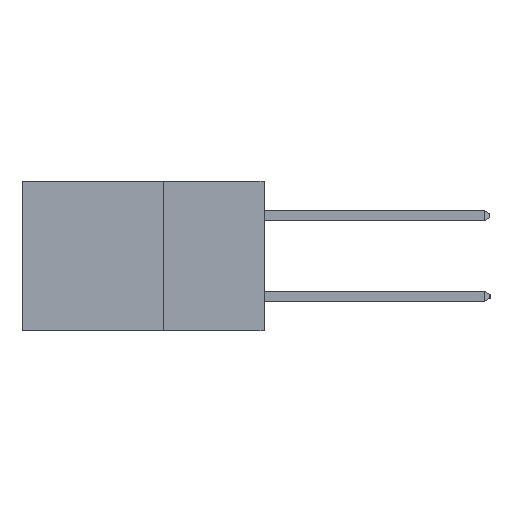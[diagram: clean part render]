
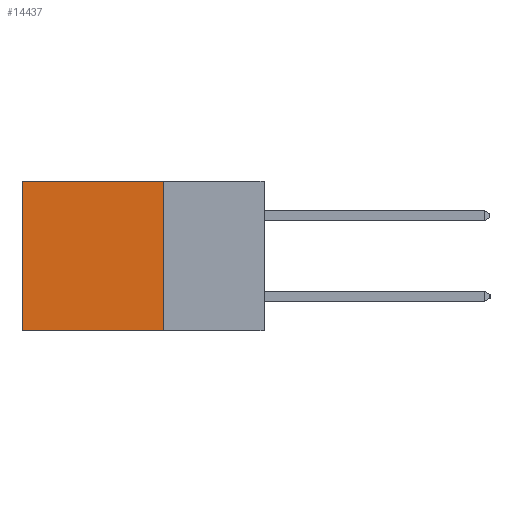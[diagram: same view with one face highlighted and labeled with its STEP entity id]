
A CAD part, left-side view. The second image highlights one B-rep face of the part: STEP entity #14437.
In plain terms, the highlighted planar face has unit normal (-1, 0, 0).
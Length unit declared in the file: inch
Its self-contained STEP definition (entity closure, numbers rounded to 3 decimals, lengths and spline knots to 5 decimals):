
#25 = CARTESIAN_POINT ( 'NONE',  ( 0.2615, 0.6, -0.37 ) ) ;
#423 = CARTESIAN_POINT ( 'NONE',  ( 0.2615, 0.25, -0.37 ) ) ;
#517 = LINE ( 'NONE', #7337, #4212 ) ;
#1311 = DIRECTION ( 'NONE',  ( 0., 0., -1. ) ) ;
#1499 = EDGE_CURVE ( 'NONE', #7244, #8643, #13840, .T. ) ;
#2924 = ORIENTED_EDGE ( 'NONE', *, *, #10534, .T. ) ;
#2953 = CARTESIAN_POINT ( 'NONE',  ( 0.2615, 0.25, -0.37 ) ) ;
#4212 = VECTOR ( 'NONE', #8859, 39.37008 ) ;
#4446 = DIRECTION ( 'NONE',  ( 0., 1., 0. ) ) ;
#4519 = CARTESIAN_POINT ( 'NONE',  ( 0.2615, 0.25, -0.37 ) ) ;
#5014 = EDGE_CURVE ( 'NONE', #8643, #6902, #14692, .T. ) ;
#5090 = DIRECTION ( 'NONE',  ( 0., 0., -1. ) ) ;
#5099 = ORIENTED_EDGE ( 'NONE', *, *, #1499, .F. ) ;
#6902 = VERTEX_POINT ( 'NONE', #25 ) ;
#7244 = VERTEX_POINT ( 'NONE', #15902 ) ;
#7337 = CARTESIAN_POINT ( 'NONE',  ( 0.2615, 0.6, -0.37 ) ) ;
#7911 = VERTEX_POINT ( 'NONE', #18838 ) ;
#7979 = VECTOR ( 'NONE', #13532, 39.37008 ) ;
#8643 = VERTEX_POINT ( 'NONE', #10597 ) ;
#8859 = DIRECTION ( 'NONE',  ( 0., 0., -1. ) ) ;
#9111 = FACE_OUTER_BOUND ( 'NONE', #16876, .T. ) ;
#9502 = ORIENTED_EDGE ( 'NONE', *, *, #16968, .T. ) ;
#9568 = PLANE ( 'NONE',  #9712 ) ;
#9712 = AXIS2_PLACEMENT_3D ( 'NONE', #423, #14033, #5090 ) ;
#10534 = EDGE_CURVE ( 'NONE', #7244, #7911, #15904, .T. ) ;
#10597 = CARTESIAN_POINT ( 'NONE',  ( 0.2615, 0.25, -0.37 ) ) ;
#12036 = CARTESIAN_POINT ( 'NONE',  ( 0.2615, 0.25, 0. ) ) ;
#13532 = DIRECTION ( 'NONE',  ( 0., 1., 0. ) ) ;
#13633 = ORIENTED_EDGE ( 'NONE', *, *, #5014, .F. ) ;
#13840 = LINE ( 'NONE', #2953, #17318 ) ;
#14033 = DIRECTION ( 'NONE',  ( 1., 0., 0. ) ) ;
#14208 = VECTOR ( 'NONE', #4446, 39.37008 ) ;
#14437 = ADVANCED_FACE ( 'NONE', ( #9111 ), #9568, .F. ) ;
#14692 = LINE ( 'NONE', #4519, #14208 ) ;
#15902 = CARTESIAN_POINT ( 'NONE',  ( 0.2615, 0.25, 0. ) ) ;
#15904 = LINE ( 'NONE', #12036, #7979 ) ;
#16876 = EDGE_LOOP ( 'NONE', ( #9502, #13633, #5099, #2924 ) ) ;
#16968 = EDGE_CURVE ( 'NONE', #7911, #6902, #517, .T. ) ;
#17318 = VECTOR ( 'NONE', #1311, 39.37008 ) ;
#18838 = CARTESIAN_POINT ( 'NONE',  ( 0.2615, 0.6, 0. ) ) ;
